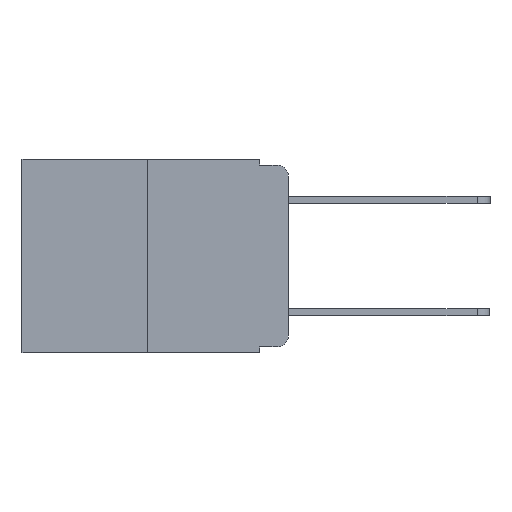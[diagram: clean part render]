
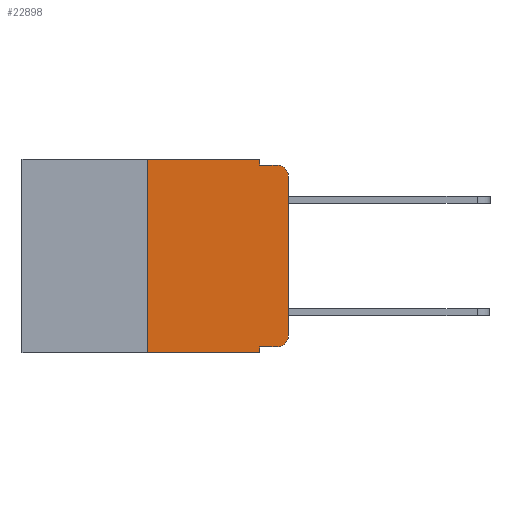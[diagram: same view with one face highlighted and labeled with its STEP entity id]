
A CAD part, left-side view. The second image highlights one B-rep face of the part: STEP entity #22898.
In plain terms, the highlighted planar face has unit normal (-1, 0, 0).
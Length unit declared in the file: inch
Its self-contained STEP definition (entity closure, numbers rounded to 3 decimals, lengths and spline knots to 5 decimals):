
#8 = AXIS2_PLACEMENT_3D ( 'NONE', #4510, #16903, #6317 ) ;
#172 = ORIENTED_EDGE ( 'NONE', *, *, #16081, .T. ) ;
#323 = VERTEX_POINT ( 'NONE', #3881 ) ;
#592 = DIRECTION ( 'NONE',  ( 0., -1., 0. ) ) ;
#760 = ORIENTED_EDGE ( 'NONE', *, *, #21466, .F. ) ;
#943 = CARTESIAN_POINT ( 'NONE',  ( 0., 0.25, 0. ) ) ;
#1274 = VECTOR ( 'NONE', #14600, 39.37008 ) ;
#1945 = CARTESIAN_POINT ( 'NONE',  ( 0., 0.051, 0. ) ) ;
#2617 = PLANE ( 'NONE',  #8 ) ;
#2782 = CARTESIAN_POINT ( 'NONE',  ( 0., 0.02, -0.03 ) ) ;
#3431 = ORIENTED_EDGE ( 'NONE', *, *, #17573, .F. ) ;
#3476 = DIRECTION ( 'NONE',  ( 0., 0., -1. ) ) ;
#3700 = EDGE_CURVE ( 'NONE', #11459, #18565, #18452, .T. ) ;
#3767 = LINE ( 'NONE', #3790, #17395 ) ;
#3790 = CARTESIAN_POINT ( 'NONE',  ( 0., 0.051, -0.01 ) ) ;
#3881 = CARTESIAN_POINT ( 'NONE',  ( 0., 0.051, -0.343 ) ) ;
#3913 = CARTESIAN_POINT ( 'NONE',  ( 0., 0.051, 0. ) ) ;
#4336 = VECTOR ( 'NONE', #17452, 39.37008 ) ;
#4492 = CARTESIAN_POINT ( 'NONE',  ( 0., 0.473, -0.343 ) ) ;
#4510 = CARTESIAN_POINT ( 'NONE',  ( 0., 0.473, 0. ) ) ;
#4881 = ORIENTED_EDGE ( 'NONE', *, *, #5280, .T. ) ;
#4909 = LINE ( 'NONE', #6890, #4336 ) ;
#5105 = DIRECTION ( 'NONE',  ( -1., 0., 0. ) ) ;
#5280 = EDGE_CURVE ( 'NONE', #21104, #17880, #20783, .T. ) ;
#5985 = VERTEX_POINT ( 'NONE', #17565 ) ;
#6186 = DIRECTION ( 'NONE',  ( 0., 0., 1. ) ) ;
#6317 = DIRECTION ( 'NONE',  ( 0., 0., -1. ) ) ;
#6881 = VECTOR ( 'NONE', #14535, 39.37008 ) ;
#6890 = CARTESIAN_POINT ( 'NONE',  ( 0., 0.051, -0.333 ) ) ;
#6893 = CARTESIAN_POINT ( 'NONE',  ( 0., 0., -0.313 ) ) ;
#7148 = CARTESIAN_POINT ( 'NONE',  ( 0., 0.25, 0. ) ) ;
#7152 = ORIENTED_EDGE ( 'NONE', *, *, #11702, .F. ) ;
#7462 = DIRECTION ( 'NONE',  ( 0., -1., 0. ) ) ;
#8131 = EDGE_CURVE ( 'NONE', #14563, #19890, #9506, .T. ) ;
#8216 = CARTESIAN_POINT ( 'NONE',  ( 0., 0., -0.03 ) ) ;
#8551 = ORIENTED_EDGE ( 'NONE', *, *, #18309, .T. ) ;
#8674 = CARTESIAN_POINT ( 'NONE',  ( 0., 0.02, -0.333 ) ) ;
#8836 = ORIENTED_EDGE ( 'NONE', *, *, #8131, .F. ) ;
#9013 = VERTEX_POINT ( 'NONE', #14353 ) ;
#9098 = DIRECTION ( 'NONE',  ( 0., 0., -1. ) ) ;
#9506 = LINE ( 'NONE', #943, #13635 ) ;
#10166 = DIRECTION ( 'NONE',  ( 0., 0., 1. ) ) ;
#11459 = VERTEX_POINT ( 'NONE', #8674 ) ;
#11686 = DIRECTION ( 'NONE',  ( -1., 0., 0. ) ) ;
#11702 = EDGE_CURVE ( 'NONE', #5985, #13125, #15079, .T. ) ;
#12067 = VECTOR ( 'NONE', #6186, 39.37008 ) ;
#12174 = ORIENTED_EDGE ( 'NONE', *, *, #3700, .T. ) ;
#12180 = DIRECTION ( 'NONE',  ( 0., -1., 0. ) ) ;
#12278 = CARTESIAN_POINT ( 'NONE',  ( 0., 0.25, -0.343 ) ) ;
#12408 = AXIS2_PLACEMENT_3D ( 'NONE', #2782, #5105, #9098 ) ;
#13119 = AXIS2_PLACEMENT_3D ( 'NONE', #13306, #11686, #3476 ) ;
#13125 = VERTEX_POINT ( 'NONE', #13422 ) ;
#13263 = VECTOR ( 'NONE', #592, 39.37008 ) ;
#13306 = CARTESIAN_POINT ( 'NONE',  ( 0., 0.02, -0.313 ) ) ;
#13422 = CARTESIAN_POINT ( 'NONE',  ( 0., 0.051, -0.01 ) ) ;
#13635 = VECTOR ( 'NONE', #10166, 39.37008 ) ;
#14353 = CARTESIAN_POINT ( 'NONE',  ( 0., 0.051, -0.333 ) ) ;
#14535 = DIRECTION ( 'NONE',  ( 0., 0., -1. ) ) ;
#14563 = VERTEX_POINT ( 'NONE', #12278 ) ;
#14600 = DIRECTION ( 'NONE',  ( 0., 0., -1. ) ) ;
#14885 = ORIENTED_EDGE ( 'NONE', *, *, #15196, .F. ) ;
#15079 = LINE ( 'NONE', #3913, #1274 ) ;
#15155 = EDGE_LOOP ( 'NONE', ( #8551, #4881, #14885, #7152, #3431, #8836, #172, #760, #15722, #12174 ) ) ;
#15196 = EDGE_CURVE ( 'NONE', #13125, #17880, #3767, .T. ) ;
#15649 = EDGE_CURVE ( 'NONE', #9013, #11459, #4909, .T. ) ;
#15722 = ORIENTED_EDGE ( 'NONE', *, *, #15649, .T. ) ;
#16081 = EDGE_CURVE ( 'NONE', #14563, #323, #21948, .T. ) ;
#16170 = LINE ( 'NONE', #18541, #12067 ) ;
#16903 = DIRECTION ( 'NONE',  ( 1., 0., 0. ) ) ;
#17395 = VECTOR ( 'NONE', #7462, 39.37008 ) ;
#17452 = DIRECTION ( 'NONE',  ( 0., -1., 0. ) ) ;
#17565 = CARTESIAN_POINT ( 'NONE',  ( 0., 0.051, 0. ) ) ;
#17573 = EDGE_CURVE ( 'NONE', #19890, #5985, #18124, .T. ) ;
#17579 = VECTOR ( 'NONE', #12180, 39.37008 ) ;
#17880 = VERTEX_POINT ( 'NONE', #19081 ) ;
#18124 = LINE ( 'NONE', #22664, #17579 ) ;
#18309 = EDGE_CURVE ( 'NONE', #18565, #21104, #16170, .T. ) ;
#18452 = CIRCLE ( 'NONE', #13119, 0.02 ) ;
#18541 = CARTESIAN_POINT ( 'NONE',  ( 0., 0., 0. ) ) ;
#18565 = VERTEX_POINT ( 'NONE', #6893 ) ;
#19081 = CARTESIAN_POINT ( 'NONE',  ( 0., 0.02, -0.01 ) ) ;
#19890 = VERTEX_POINT ( 'NONE', #7148 ) ;
#19999 = FACE_OUTER_BOUND ( 'NONE', #15155, .T. ) ;
#20326 = LINE ( 'NONE', #1945, #6881 ) ;
#20783 = CIRCLE ( 'NONE', #12408, 0.02 ) ;
#21104 = VERTEX_POINT ( 'NONE', #8216 ) ;
#21466 = EDGE_CURVE ( 'NONE', #9013, #323, #20326, .T. ) ;
#21948 = LINE ( 'NONE', #4492, #13263 ) ;
#22664 = CARTESIAN_POINT ( 'NONE',  ( 0., 0.473, 0. ) ) ;
#22898 = ADVANCED_FACE ( 'NONE', ( #19999 ), #2617, .F. ) ;
